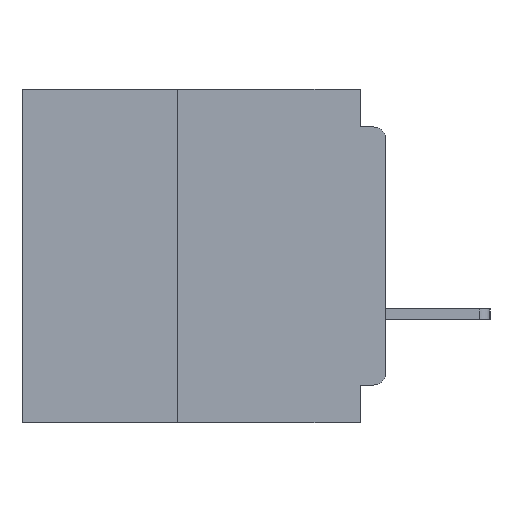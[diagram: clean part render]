
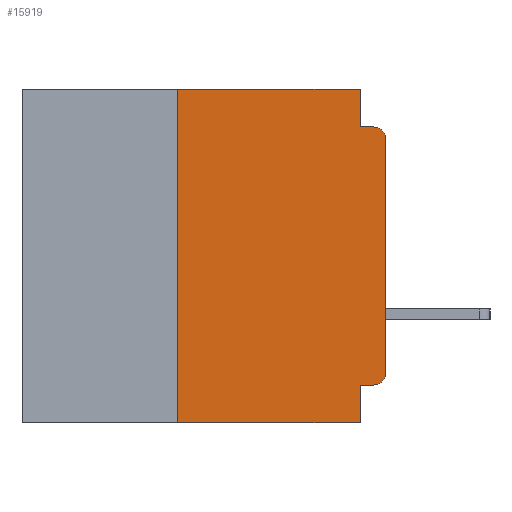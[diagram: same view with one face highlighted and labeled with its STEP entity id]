
A CAD part, left-side view. The second image highlights one B-rep face of the part: STEP entity #15919.
In plain terms, the highlighted planar face has unit normal (-1, 0, 0).
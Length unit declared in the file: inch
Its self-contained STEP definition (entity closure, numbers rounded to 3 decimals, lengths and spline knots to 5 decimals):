
#304 = CARTESIAN_POINT ( 'NONE',  ( 0., 0.031, 0. ) ) ;
#1868 = LINE ( 'NONE', #24533, #38212 ) ;
#1936 = VECTOR ( 'NONE', #44873, 39.37008 ) ;
#2139 = CARTESIAN_POINT ( 'NONE',  ( 0., 0., -0.06 ) ) ;
#2193 = CARTESIAN_POINT ( 'NONE',  ( 0., 0.015, -0.045 ) ) ;
#3050 = ORIENTED_EDGE ( 'NONE', *, *, #48624, .F. ) ;
#3369 = CARTESIAN_POINT ( 'NONE',  ( 0., 0.25, -0.4 ) ) ;
#3567 = VECTOR ( 'NONE', #59557, 39.37008 ) ;
#4073 = LINE ( 'NONE', #21135, #13745 ) ;
#5153 = VERTEX_POINT ( 'NONE', #2193 ) ;
#6095 = ORIENTED_EDGE ( 'NONE', *, *, #13747, .T. ) ;
#6259 = CARTESIAN_POINT ( 'NONE',  ( 0., 0.015, -0.34 ) ) ;
#9428 = VERTEX_POINT ( 'NONE', #40026 ) ;
#11029 = DIRECTION ( 'NONE',  ( 0., 0., -1. ) ) ;
#12797 = EDGE_CURVE ( 'NONE', #14095, #26553, #16700, .T. ) ;
#13089 = VERTEX_POINT ( 'NONE', #2139 ) ;
#13333 = CIRCLE ( 'NONE', #41629, 0.015 ) ;
#13745 = VECTOR ( 'NONE', #58890, 39.37008 ) ;
#13747 = EDGE_CURVE ( 'NONE', #9428, #13089, #53850, .T. ) ;
#14095 = VERTEX_POINT ( 'NONE', #17205 ) ;
#14551 = DIRECTION ( 'NONE',  ( -1., 0., 0. ) ) ;
#15090 = EDGE_CURVE ( 'NONE', #15381, #30861, #1868, .T. ) ;
#15381 = VERTEX_POINT ( 'NONE', #3369 ) ;
#15878 = ORIENTED_EDGE ( 'NONE', *, *, #17311, .T. ) ;
#15919 = ADVANCED_FACE ( 'NONE', ( #53553 ), #50007, .F. ) ;
#16658 = EDGE_LOOP ( 'NONE', ( #6095, #15878, #47657, #28131, #28288, #37066, #35952, #3050, #38302, #44189 ) ) ;
#16700 = LINE ( 'NONE', #304, #16823 ) ;
#16823 = VECTOR ( 'NONE', #33462, 39.37008 ) ;
#17163 = EDGE_CURVE ( 'NONE', #20616, #40189, #43159, .T. ) ;
#17205 = CARTESIAN_POINT ( 'NONE',  ( 0., 0.031, 0. ) ) ;
#17311 = EDGE_CURVE ( 'NONE', #13089, #5153, #57882, .T. ) ;
#19105 = VECTOR ( 'NONE', #53669, 39.37008 ) ;
#19282 = VERTEX_POINT ( 'NONE', #43220 ) ;
#19779 = DIRECTION ( 'NONE',  ( 0., 0., 1. ) ) ;
#20616 = VERTEX_POINT ( 'NONE', #37419 ) ;
#21135 = CARTESIAN_POINT ( 'NONE',  ( 0., 0.437, 0. ) ) ;
#23054 = AXIS2_PLACEMENT_3D ( 'NONE', #40537, #54772, #26507 ) ;
#23727 = VECTOR ( 'NONE', #45956, 39.37008 ) ;
#23976 = EDGE_CURVE ( 'NONE', #15381, #19282, #51770, .T. ) ;
#24533 = CARTESIAN_POINT ( 'NONE',  ( 0., 0.25, -0.4 ) ) ;
#26507 = DIRECTION ( 'NONE',  ( 0., 0., -1. ) ) ;
#26553 = VERTEX_POINT ( 'NONE', #44816 ) ;
#27204 = LINE ( 'NONE', #39908, #1936 ) ;
#28131 = ORIENTED_EDGE ( 'NONE', *, *, #12797, .F. ) ;
#28288 = ORIENTED_EDGE ( 'NONE', *, *, #38977, .F. ) ;
#30861 = VERTEX_POINT ( 'NONE', #42179 ) ;
#31299 = CARTESIAN_POINT ( 'NONE',  ( 0., 0., 0. ) ) ;
#31925 = DIRECTION ( 'NONE',  ( 0., 1., 0. ) ) ;
#33462 = DIRECTION ( 'NONE',  ( 0., 0., -1. ) ) ;
#34201 = CARTESIAN_POINT ( 'NONE',  ( 0., 0.031, -0.355 ) ) ;
#35952 = ORIENTED_EDGE ( 'NONE', *, *, #23976, .T. ) ;
#36720 = CARTESIAN_POINT ( 'NONE',  ( 0., 0., -0.355 ) ) ;
#37066 = ORIENTED_EDGE ( 'NONE', *, *, #15090, .F. ) ;
#37242 = EDGE_CURVE ( 'NONE', #26553, #5153, #27204, .T. ) ;
#37419 = CARTESIAN_POINT ( 'NONE',  ( 0., 0.015, -0.355 ) ) ;
#38212 = VECTOR ( 'NONE', #19779, 39.37008 ) ;
#38302 = ORIENTED_EDGE ( 'NONE', *, *, #17163, .F. ) ;
#38977 = EDGE_CURVE ( 'NONE', #30861, #14095, #4073, .T. ) ;
#39364 = DIRECTION ( 'NONE',  ( -1., 0., 0. ) ) ;
#39908 = CARTESIAN_POINT ( 'NONE',  ( 0., 0., -0.045 ) ) ;
#40026 = CARTESIAN_POINT ( 'NONE',  ( 0., 0., -0.34 ) ) ;
#40189 = VERTEX_POINT ( 'NONE', #34201 ) ;
#40537 = CARTESIAN_POINT ( 'NONE',  ( 0., 0.437, 0. ) ) ;
#41218 = CARTESIAN_POINT ( 'NONE',  ( 0., 0.437, -0.4 ) ) ;
#41629 = AXIS2_PLACEMENT_3D ( 'NONE', #6259, #39364, #11029 ) ;
#41979 = EDGE_CURVE ( 'NONE', #20616, #9428, #13333, .T. ) ;
#42179 = CARTESIAN_POINT ( 'NONE',  ( 0., 0.25, 0. ) ) ;
#42833 = CARTESIAN_POINT ( 'NONE',  ( 0., 0.015, -0.06 ) ) ;
#43159 = LINE ( 'NONE', #36720, #54217 ) ;
#43220 = CARTESIAN_POINT ( 'NONE',  ( 0., 0.031, -0.4 ) ) ;
#44187 = CARTESIAN_POINT ( 'NONE',  ( 0., 0.031, -0.4 ) ) ;
#44189 = ORIENTED_EDGE ( 'NONE', *, *, #41979, .T. ) ;
#44816 = CARTESIAN_POINT ( 'NONE',  ( 0., 0.031, -0.045 ) ) ;
#44873 = DIRECTION ( 'NONE',  ( 0., -1., 0. ) ) ;
#45623 = AXIS2_PLACEMENT_3D ( 'NONE', #42833, #14551, #47588 ) ;
#45956 = DIRECTION ( 'NONE',  ( 0., -1., 0. ) ) ;
#47588 = DIRECTION ( 'NONE',  ( 0., 0., -1. ) ) ;
#47657 = ORIENTED_EDGE ( 'NONE', *, *, #37242, .F. ) ;
#48624 = EDGE_CURVE ( 'NONE', #40189, #19282, #55292, .T. ) ;
#50007 = PLANE ( 'NONE',  #23054 ) ;
#51770 = LINE ( 'NONE', #41218, #23727 ) ;
#53553 = FACE_OUTER_BOUND ( 'NONE', #16658, .T. ) ;
#53669 = DIRECTION ( 'NONE',  ( 0., 0., -1. ) ) ;
#53850 = LINE ( 'NONE', #31299, #3567 ) ;
#54217 = VECTOR ( 'NONE', #31925, 39.37008 ) ;
#54772 = DIRECTION ( 'NONE',  ( 1., 0., 0. ) ) ;
#55292 = LINE ( 'NONE', #44187, #19105 ) ;
#57882 = CIRCLE ( 'NONE', #45623, 0.015 ) ;
#58890 = DIRECTION ( 'NONE',  ( 0., -1., 0. ) ) ;
#59557 = DIRECTION ( 'NONE',  ( 0., 0., 1. ) ) ;
